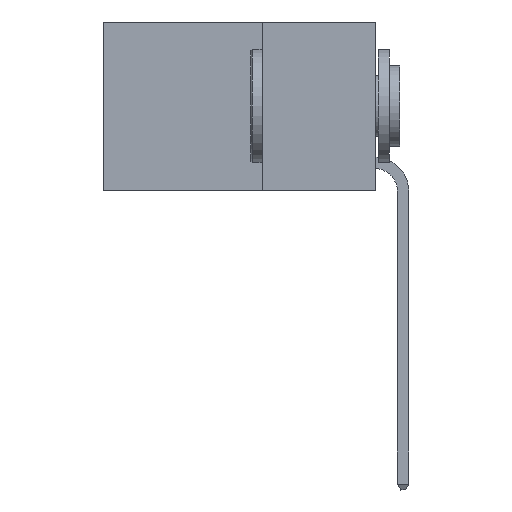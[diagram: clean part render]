
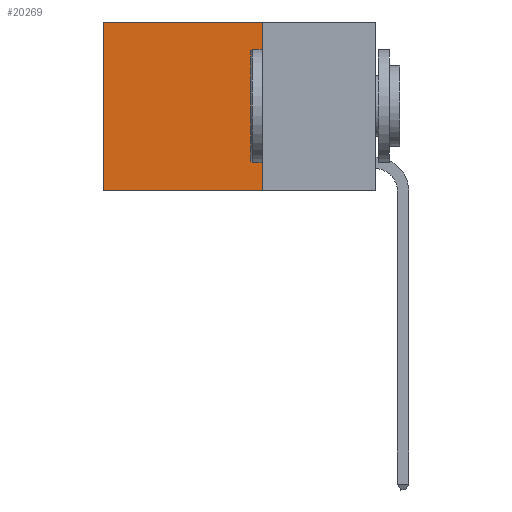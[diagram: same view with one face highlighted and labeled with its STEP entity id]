
A CAD part, left-side view. The second image highlights one B-rep face of the part: STEP entity #20269.
In plain terms, the highlighted planar face has unit normal (-1, 0, 0).
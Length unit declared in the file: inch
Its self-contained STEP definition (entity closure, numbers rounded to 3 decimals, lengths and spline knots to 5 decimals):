
#61 = LINE ( 'NONE', #5849, #10008 ) ;
#473 = LINE ( 'NONE', #16665, #16847 ) ;
#1569 = FACE_OUTER_BOUND ( 'NONE', #6127, .T. ) ;
#1760 = EDGE_CURVE ( 'NONE', #14847, #15385, #21383, .T. ) ;
#1777 = VERTEX_POINT ( 'NONE', #8514 ) ;
#2672 = DIRECTION ( 'NONE',  ( 0., 1., 0. ) ) ;
#3069 = CARTESIAN_POINT ( 'NONE',  ( 0.2625, 0.6, 0. ) ) ;
#3946 = DIRECTION ( 'NONE',  ( 0., 1., 0. ) ) ;
#4909 = CARTESIAN_POINT ( 'NONE',  ( 0.2625, 0.25, 0. ) ) ;
#5809 = VECTOR ( 'NONE', #2672, 39.37008 ) ;
#5849 = CARTESIAN_POINT ( 'NONE',  ( 0.2625, 0.25, 0. ) ) ;
#6127 = EDGE_LOOP ( 'NONE', ( #18159, #23281, #9033, #15168 ) ) ;
#6503 = EDGE_CURVE ( 'NONE', #1777, #15385, #20763, .T. ) ;
#7944 = CARTESIAN_POINT ( 'NONE',  ( 0.2625, 0.6, -0.37 ) ) ;
#8514 = CARTESIAN_POINT ( 'NONE',  ( 0.2625, 0.25, -0.37 ) ) ;
#8572 = VERTEX_POINT ( 'NONE', #13135 ) ;
#9033 = ORIENTED_EDGE ( 'NONE', *, *, #20922, .F. ) ;
#10008 = VECTOR ( 'NONE', #3946, 39.37008 ) ;
#10015 = CARTESIAN_POINT ( 'NONE',  ( 0.2625, 0.25, -0.37 ) ) ;
#12103 = DIRECTION ( 'NONE',  ( 1., 0., 0. ) ) ;
#12916 = CARTESIAN_POINT ( 'NONE',  ( 0.2625, 0.6, 0. ) ) ;
#13135 = CARTESIAN_POINT ( 'NONE',  ( 0.2625, 0.25, 0. ) ) ;
#13867 = PLANE ( 'NONE',  #14925 ) ;
#14807 = EDGE_CURVE ( 'NONE', #8572, #14847, #61, .T. ) ;
#14847 = VERTEX_POINT ( 'NONE', #12916 ) ;
#14925 = AXIS2_PLACEMENT_3D ( 'NONE', #4909, #12103, #19328 ) ;
#15117 = DIRECTION ( 'NONE',  ( 0., 0., -1. ) ) ;
#15168 = ORIENTED_EDGE ( 'NONE', *, *, #14807, .T. ) ;
#15385 = VERTEX_POINT ( 'NONE', #7944 ) ;
#16084 = VECTOR ( 'NONE', #21038, 39.37008 ) ;
#16665 = CARTESIAN_POINT ( 'NONE',  ( 0.2625, 0.25, 0. ) ) ;
#16847 = VECTOR ( 'NONE', #15117, 39.37008 ) ;
#18159 = ORIENTED_EDGE ( 'NONE', *, *, #1760, .T. ) ;
#19328 = DIRECTION ( 'NONE',  ( 0., 0., -1. ) ) ;
#20269 = ADVANCED_FACE ( 'NONE', ( #1569 ), #13867, .F. ) ;
#20763 = LINE ( 'NONE', #10015, #5809 ) ;
#20922 = EDGE_CURVE ( 'NONE', #8572, #1777, #473, .T. ) ;
#21038 = DIRECTION ( 'NONE',  ( 0., 0., -1. ) ) ;
#21383 = LINE ( 'NONE', #3069, #16084 ) ;
#23281 = ORIENTED_EDGE ( 'NONE', *, *, #6503, .F. ) ;
